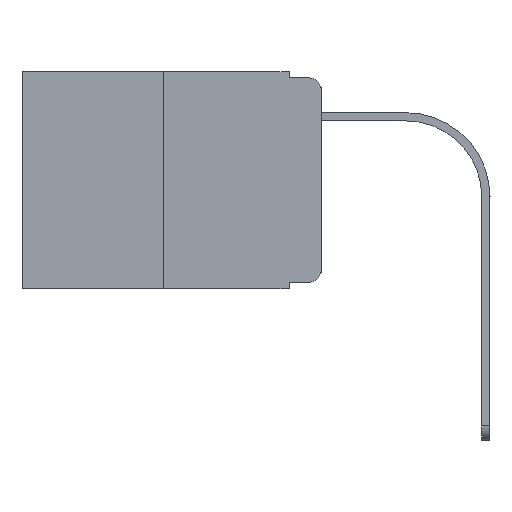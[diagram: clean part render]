
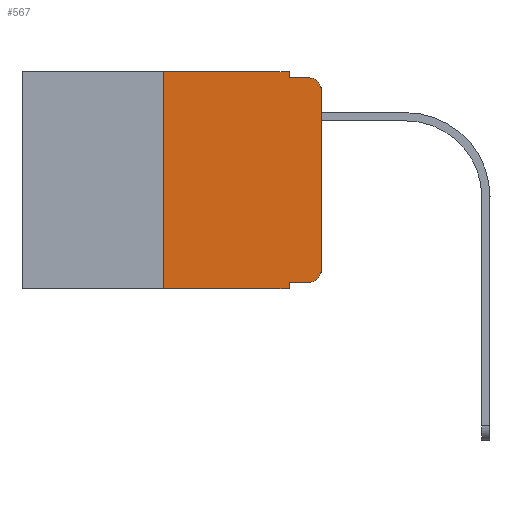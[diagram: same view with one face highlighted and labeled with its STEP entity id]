
A CAD part, left-side view. The second image highlights one B-rep face of the part: STEP entity #567.
In plain terms, the highlighted planar face has unit normal (-1, 0, 0).
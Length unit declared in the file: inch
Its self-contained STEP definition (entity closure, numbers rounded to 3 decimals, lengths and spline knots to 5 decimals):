
#79 = EDGE_CURVE ( 'NONE', #10440, #12388, #12045, .T. ) ;
#567 = ADVANCED_FACE ( 'NONE', ( #12770 ), #696, .F. ) ;
#696 = PLANE ( 'NONE',  #6919 ) ;
#912 = VECTOR ( 'NONE', #20548, 39.37008 ) ;
#1007 = DIRECTION ( 'NONE',  ( 0., 0., -1. ) ) ;
#1014 = EDGE_LOOP ( 'NONE', ( #1895, #9625, #15202, #20853, #21639, #13099, #1762, #4491, #8525, #14285 ) ) ;
#1714 = VECTOR ( 'NONE', #2110, 39.37008 ) ;
#1762 = ORIENTED_EDGE ( 'NONE', *, *, #2247, .T. ) ;
#1895 = ORIENTED_EDGE ( 'NONE', *, *, #2149, .T. ) ;
#1924 = VERTEX_POINT ( 'NONE', #5796 ) ;
#2110 = DIRECTION ( 'NONE',  ( 0., -1., 0. ) ) ;
#2149 = EDGE_CURVE ( 'NONE', #20616, #17183, #8136, .T. ) ;
#2247 = EDGE_CURVE ( 'NONE', #10440, #2319, #3474, .T. ) ;
#2312 = DIRECTION ( 'NONE',  ( -1., 0., 0. ) ) ;
#2319 = VERTEX_POINT ( 'NONE', #4003 ) ;
#2654 = CARTESIAN_POINT ( 'NONE',  ( 0., 0.051, -0.01 ) ) ;
#3255 = DIRECTION ( 'NONE',  ( 0., -1., 0. ) ) ;
#3421 = EDGE_CURVE ( 'NONE', #10634, #5041, #5246, .T. ) ;
#3474 = LINE ( 'NONE', #14992, #5158 ) ;
#4003 = CARTESIAN_POINT ( 'NONE',  ( 0., 0.051, -0.343 ) ) ;
#4221 = DIRECTION ( 'NONE',  ( 0., 0., -1. ) ) ;
#4491 = ORIENTED_EDGE ( 'NONE', *, *, #17544, .F. ) ;
#4768 = CARTESIAN_POINT ( 'NONE',  ( 0., 0.473, 0. ) ) ;
#4868 = CARTESIAN_POINT ( 'NONE',  ( 0., 0.051, 0. ) ) ;
#5041 = VERTEX_POINT ( 'NONE', #5107 ) ;
#5092 = AXIS2_PLACEMENT_3D ( 'NONE', #21235, #2312, #21123 ) ;
#5107 = CARTESIAN_POINT ( 'NONE',  ( 0., 0.02, -0.333 ) ) ;
#5158 = VECTOR ( 'NONE', #3255, 39.37008 ) ;
#5194 = EDGE_CURVE ( 'NONE', #1924, #16104, #17725, .T. ) ;
#5246 = LINE ( 'NONE', #12003, #20014 ) ;
#5317 = CARTESIAN_POINT ( 'NONE',  ( 0., 0.051, -0.01 ) ) ;
#5532 = EDGE_CURVE ( 'NONE', #5041, #20616, #21349, .T. ) ;
#5543 = CARTESIAN_POINT ( 'NONE',  ( 0., 0., -0.313 ) ) ;
#5796 = CARTESIAN_POINT ( 'NONE',  ( 0., 0.051, 0. ) ) ;
#6275 = VECTOR ( 'NONE', #4221, 39.37008 ) ;
#6624 = EDGE_CURVE ( 'NONE', #12388, #1924, #16829, .T. ) ;
#6919 = AXIS2_PLACEMENT_3D ( 'NONE', #18871, #11215, #12658 ) ;
#7638 = CARTESIAN_POINT ( 'NONE',  ( 0., 0.02, -0.03 ) ) ;
#8136 = LINE ( 'NONE', #11348, #13755 ) ;
#8525 = ORIENTED_EDGE ( 'NONE', *, *, #3421, .T. ) ;
#8725 = CARTESIAN_POINT ( 'NONE',  ( 0., 0.25, 0. ) ) ;
#9434 = CARTESIAN_POINT ( 'NONE',  ( 0., 0.051, 0. ) ) ;
#9567 = VERTEX_POINT ( 'NONE', #19180 ) ;
#9625 = ORIENTED_EDGE ( 'NONE', *, *, #11608, .T. ) ;
#9682 = DIRECTION ( 'NONE',  ( 0., 0., 1. ) ) ;
#10302 = LINE ( 'NONE', #5317, #1714 ) ;
#10440 = VERTEX_POINT ( 'NONE', #11155 ) ;
#10628 = DIRECTION ( 'NONE',  ( -1., 0., 0. ) ) ;
#10634 = VERTEX_POINT ( 'NONE', #18870 ) ;
#11155 = CARTESIAN_POINT ( 'NONE',  ( 0., 0.25, -0.343 ) ) ;
#11215 = DIRECTION ( 'NONE',  ( 1., 0., 0. ) ) ;
#11348 = CARTESIAN_POINT ( 'NONE',  ( 0., 0., 0. ) ) ;
#11559 = AXIS2_PLACEMENT_3D ( 'NONE', #7638, #10628, #1007 ) ;
#11608 = EDGE_CURVE ( 'NONE', #17183, #9567, #14014, .T. ) ;
#11631 = DIRECTION ( 'NONE',  ( 0., 0., -1. ) ) ;
#12003 = CARTESIAN_POINT ( 'NONE',  ( 0., 0.051, -0.333 ) ) ;
#12045 = LINE ( 'NONE', #8725, #912 ) ;
#12388 = VERTEX_POINT ( 'NONE', #21259 ) ;
#12658 = DIRECTION ( 'NONE',  ( 0., 0., -1. ) ) ;
#12770 = FACE_OUTER_BOUND ( 'NONE', #1014, .T. ) ;
#13099 = ORIENTED_EDGE ( 'NONE', *, *, #79, .F. ) ;
#13755 = VECTOR ( 'NONE', #9682, 39.37008 ) ;
#13927 = EDGE_CURVE ( 'NONE', #16104, #9567, #10302, .T. ) ;
#14014 = CIRCLE ( 'NONE', #11559, 0.02 ) ;
#14285 = ORIENTED_EDGE ( 'NONE', *, *, #5532, .T. ) ;
#14992 = CARTESIAN_POINT ( 'NONE',  ( 0., 0.473, -0.343 ) ) ;
#15202 = ORIENTED_EDGE ( 'NONE', *, *, #13927, .F. ) ;
#15655 = VECTOR ( 'NONE', #21683, 39.37008 ) ;
#15827 = CARTESIAN_POINT ( 'NONE',  ( 0., 0., -0.03 ) ) ;
#16104 = VERTEX_POINT ( 'NONE', #2654 ) ;
#16829 = LINE ( 'NONE', #4768, #15655 ) ;
#17183 = VERTEX_POINT ( 'NONE', #15827 ) ;
#17544 = EDGE_CURVE ( 'NONE', #10634, #2319, #20027, .T. ) ;
#17663 = VECTOR ( 'NONE', #11631, 39.37008 ) ;
#17725 = LINE ( 'NONE', #9434, #6275 ) ;
#18870 = CARTESIAN_POINT ( 'NONE',  ( 0., 0.051, -0.333 ) ) ;
#18871 = CARTESIAN_POINT ( 'NONE',  ( 0., 0.473, 0. ) ) ;
#19180 = CARTESIAN_POINT ( 'NONE',  ( 0., 0.02, -0.01 ) ) ;
#20014 = VECTOR ( 'NONE', #20829, 39.37008 ) ;
#20027 = LINE ( 'NONE', #4868, #17663 ) ;
#20548 = DIRECTION ( 'NONE',  ( 0., 0., 1. ) ) ;
#20616 = VERTEX_POINT ( 'NONE', #5543 ) ;
#20829 = DIRECTION ( 'NONE',  ( 0., -1., 0. ) ) ;
#20853 = ORIENTED_EDGE ( 'NONE', *, *, #5194, .F. ) ;
#21123 = DIRECTION ( 'NONE',  ( 0., 0., -1. ) ) ;
#21235 = CARTESIAN_POINT ( 'NONE',  ( 0., 0.02, -0.313 ) ) ;
#21259 = CARTESIAN_POINT ( 'NONE',  ( 0., 0.25, 0. ) ) ;
#21349 = CIRCLE ( 'NONE', #5092, 0.02 ) ;
#21639 = ORIENTED_EDGE ( 'NONE', *, *, #6624, .F. ) ;
#21683 = DIRECTION ( 'NONE',  ( 0., -1., 0. ) ) ;
